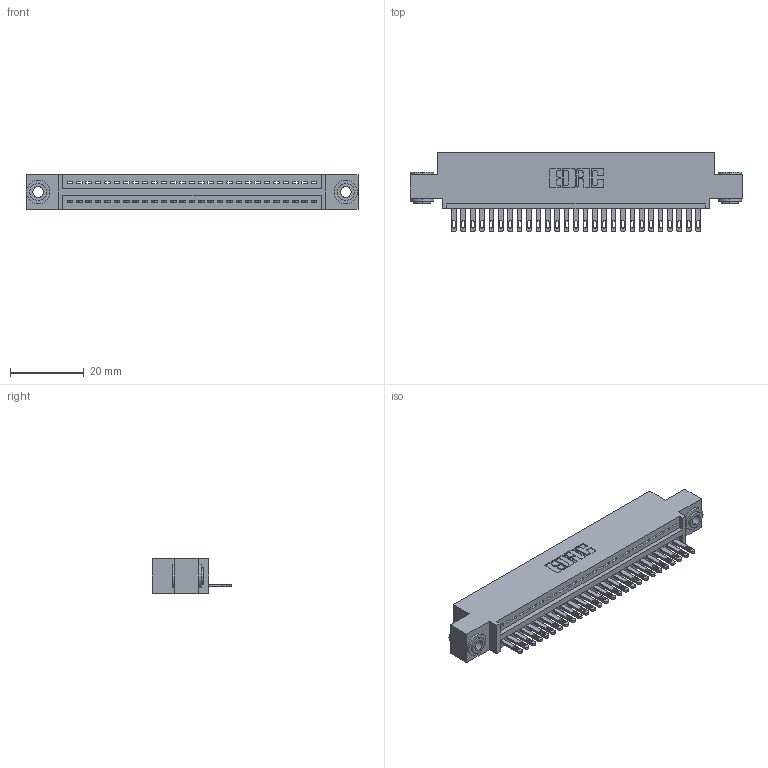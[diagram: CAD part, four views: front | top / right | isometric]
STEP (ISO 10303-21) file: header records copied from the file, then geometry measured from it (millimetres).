
FILE_DESCRIPTION (( 'STEP AP203' ), '1' );
FILE_NAME ('895-027-500-403.STEP', '2020-09-25T15:24:14', ( '' ), ( '' ), 'SwSTEP 2.0', 'SolidWorks 2020', '' );
FILE_SCHEMA (( 'CONFIG_CONTROL_DESIGN' ));
Length unit declared in the file: inch
Products named in the file (4): 845 Part_0.110 Offset - 0.156 Dia-TH; 345-250-002_345-250-002-102; 345-292-001_345-293-100; 895-027-500-403
Assembly tree (30 placements, depth 2):
  895-027-500-403
    845 Part_0.110 Offset - 0.156 Dia-TH
    345-292-001_345-293-100  x27
    345-250-002_345-250-002-102  x2
Bounding box: 89.79 x 21.51 x 9.4 mm (x, y, z)
Volume: 8368.1 mm3; surface area: 11273.6 mm2
Topology: 30 solids, 30 shells, 1626 faces, 4965 edges, 3306 vertices
Faces by surface type: plane 1012, cylinder 606, cone 8
Entity records: 23052 total; most frequent: CARTESIAN_POINT 3972, ORIENTED_EDGE 3926, DIRECTION 3523, EDGE_CURVE 1963, VECTOR 1695, LINE 1695, VERTEX_POINT 1306, AXIS2_PLACEMENT_3D 914
